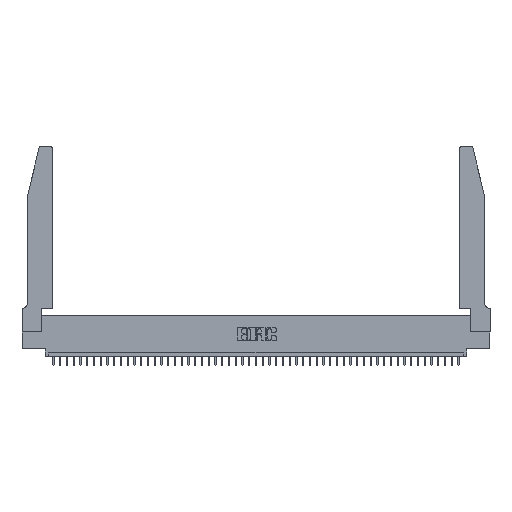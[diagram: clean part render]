
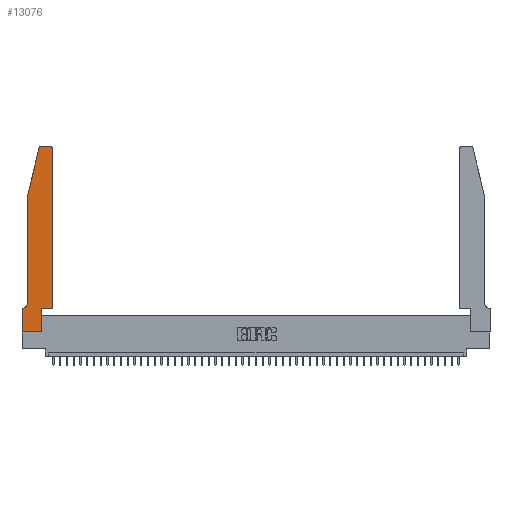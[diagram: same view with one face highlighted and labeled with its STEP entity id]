
A CAD part, top view. The second image highlights one B-rep face of the part: STEP entity #13076.
In plain terms, the highlighted planar face has unit normal (0, 0, 1).
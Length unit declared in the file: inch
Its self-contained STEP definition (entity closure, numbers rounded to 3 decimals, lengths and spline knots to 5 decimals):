
#296 = VERTEX_POINT ( 'NONE', #9352 ) ;
#348 = VECTOR ( 'NONE', #5672, 39.37008 ) ;
#366 = LINE ( 'NONE', #27227, #3861 ) ;
#417 = EDGE_CURVE ( 'NONE', #31508, #8711, #17416, .T. ) ;
#831 = DIRECTION ( 'NONE',  ( -1., 0., 0. ) ) ;
#1481 = EDGE_CURVE ( 'NONE', #24999, #31508, #15997, .T. ) ;
#3462 = CARTESIAN_POINT ( 'NONE',  ( 0., 0., 0.37 ) ) ;
#3747 = AXIS2_PLACEMENT_3D ( 'NONE', #26087, #45414, #3884 ) ;
#3858 = DIRECTION ( 'NONE',  ( 0., 0., 1. ) ) ;
#3861 = VECTOR ( 'NONE', #12353, 39.37008 ) ;
#3884 = DIRECTION ( 'NONE',  ( 1., 0., 0. ) ) ;
#5055 = VERTEX_POINT ( 'NONE', #26060 ) ;
#5672 = DIRECTION ( 'NONE',  ( 0., 1., 0. ) ) ;
#5820 = EDGE_LOOP ( 'NONE', ( #14340, #15625, #11353, #31034, #16361, #21996, #26911, #5892, #6725, #7218, #18918, #15691 ) ) ;
#5892 = ORIENTED_EDGE ( 'NONE', *, *, #22029, .T. ) ;
#6030 = DIRECTION ( 'NONE',  ( -1., 0., 0. ) ) ;
#6572 = CARTESIAN_POINT ( 'NONE',  ( 0., 0.35, 0.37 ) ) ;
#6725 = ORIENTED_EDGE ( 'NONE', *, *, #12485, .T. ) ;
#6810 = DIRECTION ( 'NONE',  ( 1., 0., 0. ) ) ;
#7218 = ORIENTED_EDGE ( 'NONE', *, *, #16635, .T. ) ;
#8634 = EDGE_CURVE ( 'NONE', #15998, #34903, #20844, .T. ) ;
#8711 = VERTEX_POINT ( 'NONE', #3462 ) ;
#9352 = CARTESIAN_POINT ( 'NONE',  ( 0.284, 2.75, 0.37 ) ) ;
#9514 = DIRECTION ( 'NONE',  ( 1., 0., 0. ) ) ;
#9616 = AXIS2_PLACEMENT_3D ( 'NONE', #36051, #17524, #6030 ) ;
#10001 = CARTESIAN_POINT ( 'NONE',  ( 0.284, 2.72, 0.37 ) ) ;
#11182 = EDGE_CURVE ( 'NONE', #41663, #42979, #43550, .T. ) ;
#11353 = ORIENTED_EDGE ( 'NONE', *, *, #8634, .T. ) ;
#11470 = DIRECTION ( 'NONE',  ( 0., 1., 0. ) ) ;
#12353 = DIRECTION ( 'NONE',  ( 1., 0., 0. ) ) ;
#12485 = EDGE_CURVE ( 'NONE', #28800, #5055, #26926, .T. ) ;
#12487 = EDGE_CURVE ( 'NONE', #42979, #296, #35219, .T. ) ;
#13076 = ADVANCED_FACE ( 'NONE', ( #28292 ), #13671, .T. ) ;
#13442 = DIRECTION ( 'NONE',  ( 0., 0., 1. ) ) ;
#13671 = PLANE ( 'NONE',  #40174 ) ;
#14274 = EDGE_CURVE ( 'NONE', #296, #15998, #19090, .T. ) ;
#14340 = ORIENTED_EDGE ( 'NONE', *, *, #12487, .T. ) ;
#15090 = CIRCLE ( 'NONE', #9616, 0.07 ) ;
#15625 = ORIENTED_EDGE ( 'NONE', *, *, #14274, .T. ) ;
#15691 = ORIENTED_EDGE ( 'NONE', *, *, #11182, .T. ) ;
#15997 = LINE ( 'NONE', #22582, #47532 ) ;
#15998 = VERTEX_POINT ( 'NONE', #22573 ) ;
#16361 = ORIENTED_EDGE ( 'NONE', *, *, #32147, .T. ) ;
#16417 = CARTESIAN_POINT ( 'NONE',  ( 0.0755, 0.42, 0.37 ) ) ;
#16635 = EDGE_CURVE ( 'NONE', #5055, #41074, #35654, .T. ) ;
#17416 = LINE ( 'NONE', #44515, #20911 ) ;
#17524 = DIRECTION ( 'NONE',  ( 0., 0., -1. ) ) ;
#17753 = VERTEX_POINT ( 'NONE', #16417 ) ;
#18156 = CARTESIAN_POINT ( 'NONE',  ( 0., 0.35, 0.37 ) ) ;
#18918 = ORIENTED_EDGE ( 'NONE', *, *, #27224, .T. ) ;
#19090 = CIRCLE ( 'NONE', #47936, 0.03 ) ;
#20579 = CARTESIAN_POINT ( 'NONE',  ( 0.2605, 2.75, 0.37 ) ) ;
#20834 = EDGE_CURVE ( 'NONE', #34903, #17753, #41404, .T. ) ;
#20844 = LINE ( 'NONE', #35483, #26890 ) ;
#20911 = VECTOR ( 'NONE', #28617, 39.37008 ) ;
#21557 = VECTOR ( 'NONE', #35897, 39.37008 ) ;
#21996 = ORIENTED_EDGE ( 'NONE', *, *, #1481, .T. ) ;
#22029 = EDGE_CURVE ( 'NONE', #8711, #28800, #366, .T. ) ;
#22573 = CARTESIAN_POINT ( 'NONE',  ( 0.25487, 2.72718, 0.37 ) ) ;
#22582 = CARTESIAN_POINT ( 'NONE',  ( 0.0755, 0.35, 0.37 ) ) ;
#24999 = VERTEX_POINT ( 'NONE', #30888 ) ;
#26060 = CARTESIAN_POINT ( 'NONE',  ( 0.2865, 0.35, 0.37 ) ) ;
#26087 = CARTESIAN_POINT ( 'NONE',  ( 0.4205, 2.72, 0.37 ) ) ;
#26725 = CARTESIAN_POINT ( 'NONE',  ( 0.0755, 2., 0.37 ) ) ;
#26890 = VECTOR ( 'NONE', #27905, 39.37008 ) ;
#26911 = ORIENTED_EDGE ( 'NONE', *, *, #417, .T. ) ;
#26926 = LINE ( 'NONE', #42097, #348 ) ;
#27215 = DIRECTION ( 'NONE',  ( 0., -1., 0. ) ) ;
#27224 = EDGE_CURVE ( 'NONE', #41074, #41663, #44945, .T. ) ;
#27227 = CARTESIAN_POINT ( 'NONE',  ( 0., 0., 0.37 ) ) ;
#27905 = DIRECTION ( 'NONE',  ( -0.239, -0.971, 0. ) ) ;
#27931 = CARTESIAN_POINT ( 'NONE',  ( 0.4505, 0.35, 0.37 ) ) ;
#28292 = FACE_OUTER_BOUND ( 'NONE', #5820, .T. ) ;
#28617 = DIRECTION ( 'NONE',  ( 0., -1., 0. ) ) ;
#28800 = VERTEX_POINT ( 'NONE', #42519 ) ;
#30888 = CARTESIAN_POINT ( 'NONE',  ( 0.0055, 0.35, 0.37 ) ) ;
#31034 = ORIENTED_EDGE ( 'NONE', *, *, #20834, .T. ) ;
#31508 = VERTEX_POINT ( 'NONE', #18156 ) ;
#31527 = DIRECTION ( 'NONE',  ( -1., 0., 0. ) ) ;
#32147 = EDGE_CURVE ( 'NONE', #17753, #24999, #15090, .T. ) ;
#32972 = CARTESIAN_POINT ( 'NONE',  ( 0.4505, 2.72, 0.37 ) ) ;
#34903 = VERTEX_POINT ( 'NONE', #45163 ) ;
#35219 = LINE ( 'NONE', #20579, #36232 ) ;
#35483 = CARTESIAN_POINT ( 'NONE',  ( 0.0755, 2., 0.37 ) ) ;
#35654 = LINE ( 'NONE', #43741, #21557 ) ;
#35731 = VECTOR ( 'NONE', #27215, 39.37008 ) ;
#35897 = DIRECTION ( 'NONE',  ( 1., 0., 0. ) ) ;
#36051 = CARTESIAN_POINT ( 'NONE',  ( 0.0055, 0.42, 0.37 ) ) ;
#36232 = VECTOR ( 'NONE', #31527, 39.37008 ) ;
#36398 = CARTESIAN_POINT ( 'NONE',  ( 0.4505, 0.35, 0.37 ) ) ;
#40174 = AXIS2_PLACEMENT_3D ( 'NONE', #6572, #3858, #6810 ) ;
#41074 = VERTEX_POINT ( 'NONE', #27931 ) ;
#41404 = LINE ( 'NONE', #26725, #35731 ) ;
#41663 = VERTEX_POINT ( 'NONE', #32972 ) ;
#42097 = CARTESIAN_POINT ( 'NONE',  ( 0.2865, 0.35, 0.37 ) ) ;
#42519 = CARTESIAN_POINT ( 'NONE',  ( 0.2865, 0., 0.37 ) ) ;
#42979 = VERTEX_POINT ( 'NONE', #47629 ) ;
#43550 = CIRCLE ( 'NONE', #3747, 0.03 ) ;
#43741 = CARTESIAN_POINT ( 'NONE',  ( 0.4505, 0.35, 0.37 ) ) ;
#44515 = CARTESIAN_POINT ( 'NONE',  ( 0., 0., 0.37 ) ) ;
#44945 = LINE ( 'NONE', #36398, #46837 ) ;
#45163 = CARTESIAN_POINT ( 'NONE',  ( 0.0755, 2., 0.37 ) ) ;
#45414 = DIRECTION ( 'NONE',  ( 0., 0., 1. ) ) ;
#46837 = VECTOR ( 'NONE', #11470, 39.37008 ) ;
#47532 = VECTOR ( 'NONE', #831, 39.37008 ) ;
#47629 = CARTESIAN_POINT ( 'NONE',  ( 0.4205, 2.75, 0.37 ) ) ;
#47936 = AXIS2_PLACEMENT_3D ( 'NONE', #10001, #13442, #9514 ) ;
